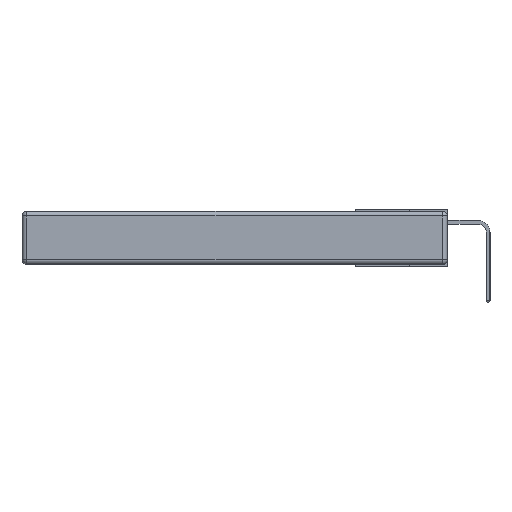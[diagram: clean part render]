
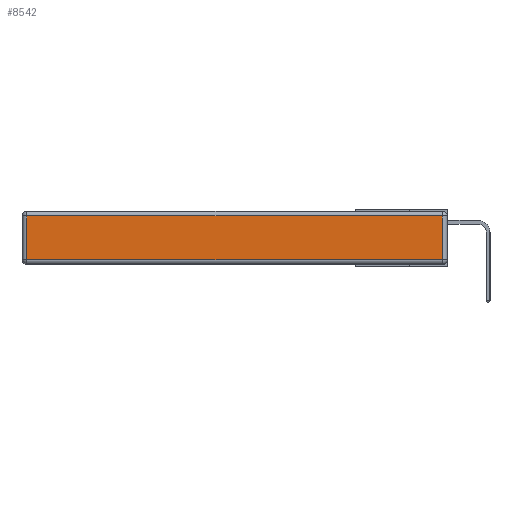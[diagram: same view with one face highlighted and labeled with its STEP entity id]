
A CAD part, left-side view. The second image highlights one B-rep face of the part: STEP entity #8542.
In plain terms, the highlighted planar face has unit normal (-1, 0, 0).
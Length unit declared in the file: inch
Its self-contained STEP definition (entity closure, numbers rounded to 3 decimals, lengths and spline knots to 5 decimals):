
#568 = CARTESIAN_POINT ( 'NONE',  ( 0., 0., -0.343 ) ) ;
#741 = VECTOR ( 'NONE', #4193, 39.37008 ) ;
#792 = EDGE_CURVE ( 'NONE', #11133, #4811, #8519, .T. ) ;
#1198 = DIRECTION ( 'NONE',  ( 0., -1., 0. ) ) ;
#1492 = PLANE ( 'NONE',  #11240 ) ;
#1714 = ORIENTED_EDGE ( 'NONE', *, *, #792, .T. ) ;
#2177 = LINE ( 'NONE', #9748, #741 ) ;
#2215 = LINE ( 'NONE', #4765, #10032 ) ;
#2282 = ORIENTED_EDGE ( 'NONE', *, *, #5515, .T. ) ;
#2612 = CARTESIAN_POINT ( 'NONE',  ( 0., 0., -0.313 ) ) ;
#2624 = ORIENTED_EDGE ( 'NONE', *, *, #6789, .T. ) ;
#2850 = CARTESIAN_POINT ( 'NONE',  ( 0., 2.72, -0.313 ) ) ;
#2987 = CARTESIAN_POINT ( 'NONE',  ( 0., 0.03, -0.313 ) ) ;
#3658 = VECTOR ( 'NONE', #1198, 39.37008 ) ;
#4138 = CARTESIAN_POINT ( 'NONE',  ( 0., 2.72, -0.343 ) ) ;
#4193 = DIRECTION ( 'NONE',  ( 0., 0., 1. ) ) ;
#4765 = CARTESIAN_POINT ( 'NONE',  ( 0., 2.75, -0.03 ) ) ;
#4811 = VERTEX_POINT ( 'NONE', #2850 ) ;
#5064 = CARTESIAN_POINT ( 'NONE',  ( 0., 0.03, -0.03 ) ) ;
#5515 = EDGE_CURVE ( 'NONE', #7326, #11133, #2215, .T. ) ;
#6490 = VERTEX_POINT ( 'NONE', #2987 ) ;
#6554 = ORIENTED_EDGE ( 'NONE', *, *, #11865, .T. ) ;
#6789 = EDGE_CURVE ( 'NONE', #6490, #7326, #2177, .T. ) ;
#6846 = LINE ( 'NONE', #2612, #3658 ) ;
#7326 = VERTEX_POINT ( 'NONE', #5064 ) ;
#7786 = FACE_OUTER_BOUND ( 'NONE', #10201, .T. ) ;
#7962 = DIRECTION ( 'NONE',  ( 0., 0., 1. ) ) ;
#8519 = LINE ( 'NONE', #4138, #10097 ) ;
#8542 = ADVANCED_FACE ( 'NONE', ( #7786 ), #1492, .T. ) ;
#9290 = DIRECTION ( 'NONE',  ( 0., 1., 0. ) ) ;
#9748 = CARTESIAN_POINT ( 'NONE',  ( 0., 0.03, -0.343 ) ) ;
#10032 = VECTOR ( 'NONE', #9290, 39.37008 ) ;
#10097 = VECTOR ( 'NONE', #10697, 39.37008 ) ;
#10201 = EDGE_LOOP ( 'NONE', ( #6554, #2624, #2282, #1714 ) ) ;
#10697 = DIRECTION ( 'NONE',  ( 0., 0., -1. ) ) ;
#10840 = CARTESIAN_POINT ( 'NONE',  ( 0., 2.72, -0.03 ) ) ;
#11133 = VERTEX_POINT ( 'NONE', #10840 ) ;
#11240 = AXIS2_PLACEMENT_3D ( 'NONE', #568, #11461, #7962 ) ;
#11461 = DIRECTION ( 'NONE',  ( -1., 0., 0. ) ) ;
#11865 = EDGE_CURVE ( 'NONE', #4811, #6490, #6846, .T. ) ;
